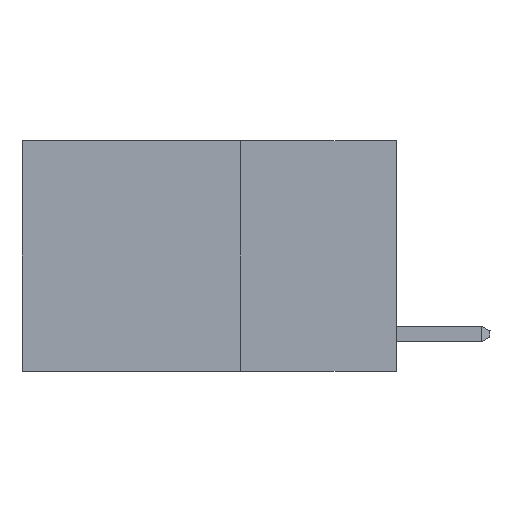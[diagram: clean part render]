
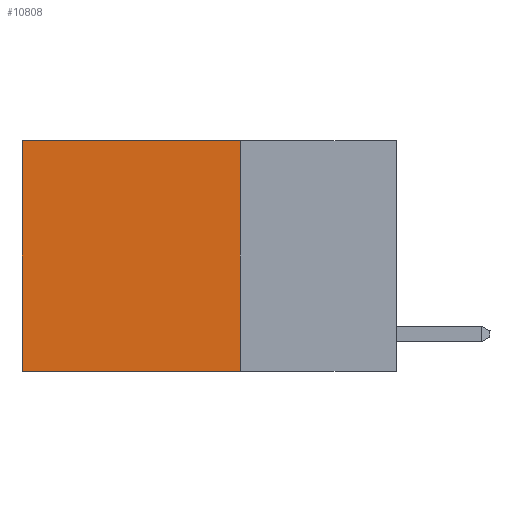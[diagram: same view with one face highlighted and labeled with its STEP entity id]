
A CAD part, left-side view. The second image highlights one B-rep face of the part: STEP entity #10808.
In plain terms, the highlighted planar face has unit normal (-1, 0, 0).
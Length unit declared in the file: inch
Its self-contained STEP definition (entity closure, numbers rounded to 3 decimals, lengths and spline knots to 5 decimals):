
#2404 = EDGE_LOOP ( 'NONE', ( #13930, #12340, #13551, #27062 ) ) ;
#4584 = DIRECTION ( 'NONE',  ( 0., 1., 0. ) ) ;
#4589 = AXIS2_PLACEMENT_3D ( 'NONE', #30115, #23038, #6291 ) ;
#6291 = DIRECTION ( 'NONE',  ( 0., 0., -1. ) ) ;
#7392 = VECTOR ( 'NONE', #7431, 39.37008 ) ;
#7431 = DIRECTION ( 'NONE',  ( 0., 0., -1. ) ) ;
#8486 = CARTESIAN_POINT ( 'NONE',  ( 0.2625, 0.25, -0.37 ) ) ;
#8894 = CARTESIAN_POINT ( 'NONE',  ( 0.2625, 0.25, 0. ) ) ;
#8956 = EDGE_CURVE ( 'NONE', #18212, #14953, #20764, .T. ) ;
#9038 = VECTOR ( 'NONE', #4584, 39.37008 ) ;
#9590 = EDGE_CURVE ( 'NONE', #25551, #17790, #11951, .T. ) ;
#10599 = CARTESIAN_POINT ( 'NONE',  ( 0.2625, 0.6, -0.37 ) ) ;
#10808 = ADVANCED_FACE ( 'NONE', ( #13631 ), #17955, .F. ) ;
#11882 = LINE ( 'NONE', #21261, #7392 ) ;
#11951 = LINE ( 'NONE', #30406, #9038 ) ;
#12340 = ORIENTED_EDGE ( 'NONE', *, *, #8956, .F. ) ;
#13551 = ORIENTED_EDGE ( 'NONE', *, *, #29604, .F. ) ;
#13631 = FACE_OUTER_BOUND ( 'NONE', #2404, .T. ) ;
#13930 = ORIENTED_EDGE ( 'NONE', *, *, #29204, .T. ) ;
#14953 = VERTEX_POINT ( 'NONE', #10599 ) ;
#14997 = CARTESIAN_POINT ( 'NONE',  ( 0.2625, 0.6, 0. ) ) ;
#15981 = DIRECTION ( 'NONE',  ( 0., 1., 0. ) ) ;
#16745 = LINE ( 'NONE', #23849, #26586 ) ;
#17790 = VERTEX_POINT ( 'NONE', #14997 ) ;
#17955 = PLANE ( 'NONE',  #4589 ) ;
#18212 = VERTEX_POINT ( 'NONE', #28998 ) ;
#20274 = VECTOR ( 'NONE', #15981, 39.37008 ) ;
#20764 = LINE ( 'NONE', #8486, #20274 ) ;
#21261 = CARTESIAN_POINT ( 'NONE',  ( 0.2625, 0.6, 0. ) ) ;
#23038 = DIRECTION ( 'NONE',  ( 1., 0., 0. ) ) ;
#23849 = CARTESIAN_POINT ( 'NONE',  ( 0.2625, 0.25, 0. ) ) ;
#25551 = VERTEX_POINT ( 'NONE', #8894 ) ;
#26321 = DIRECTION ( 'NONE',  ( 0., 0., -1. ) ) ;
#26586 = VECTOR ( 'NONE', #26321, 39.37008 ) ;
#27062 = ORIENTED_EDGE ( 'NONE', *, *, #9590, .T. ) ;
#28998 = CARTESIAN_POINT ( 'NONE',  ( 0.2625, 0.25, -0.37 ) ) ;
#29204 = EDGE_CURVE ( 'NONE', #17790, #14953, #11882, .T. ) ;
#29604 = EDGE_CURVE ( 'NONE', #25551, #18212, #16745, .T. ) ;
#30115 = CARTESIAN_POINT ( 'NONE',  ( 0.2625, 0.25, 0. ) ) ;
#30406 = CARTESIAN_POINT ( 'NONE',  ( 0.2625, 0.25, 0. ) ) ;
